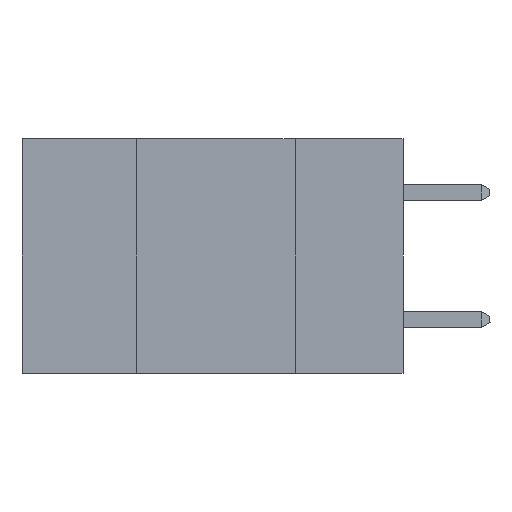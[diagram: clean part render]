
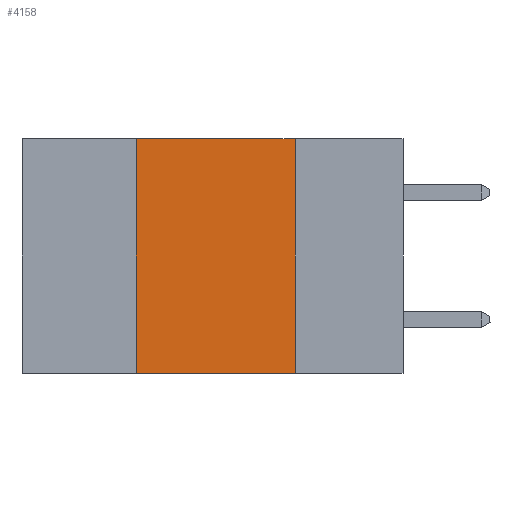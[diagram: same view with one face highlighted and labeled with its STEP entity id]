
A CAD part, left-side view. The second image highlights one B-rep face of the part: STEP entity #4158.
In plain terms, the highlighted planar face has unit normal (-1, 0, 0).
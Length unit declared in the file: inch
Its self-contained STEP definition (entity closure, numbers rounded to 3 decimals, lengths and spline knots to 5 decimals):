
#56 = VERTEX_POINT ( 'NONE', #4132 ) ;
#407 = ORIENTED_EDGE ( 'NONE', *, *, #18140, .F. ) ;
#415 = CARTESIAN_POINT ( 'NONE',  ( 0., 0.6, 0. ) ) ;
#479 = CARTESIAN_POINT ( 'NONE',  ( 0., 0.6, 0. ) ) ;
#500 = VERTEX_POINT ( 'NONE', #14114 ) ;
#1585 = LINE ( 'NONE', #24247, #8434 ) ;
#2094 = FACE_OUTER_BOUND ( 'NONE', #13984, .T. ) ;
#2759 = EDGE_CURVE ( 'NONE', #56, #4055, #1585, .T. ) ;
#3131 = CARTESIAN_POINT ( 'NONE',  ( 0., 0.17, -0.37 ) ) ;
#4055 = VERTEX_POINT ( 'NONE', #3131 ) ;
#4132 = CARTESIAN_POINT ( 'NONE',  ( 0., 0.42, -0.37 ) ) ;
#4158 = ADVANCED_FACE ( 'NONE', ( #2094 ), #17834, .F. ) ;
#6752 = EDGE_CURVE ( 'NONE', #16258, #500, #18745, .T. ) ;
#7124 = DIRECTION ( 'NONE',  ( 0., -1., 0. ) ) ;
#7333 = VECTOR ( 'NONE', #21498, 39.37008 ) ;
#8434 = VECTOR ( 'NONE', #7124, 39.37008 ) ;
#8459 = DIRECTION ( 'NONE',  ( 1., 0., 0. ) ) ;
#10269 = ORIENTED_EDGE ( 'NONE', *, *, #6752, .F. ) ;
#11099 = ORIENTED_EDGE ( 'NONE', *, *, #18207, .F. ) ;
#11165 = CARTESIAN_POINT ( 'NONE',  ( 0., 0.42, 0. ) ) ;
#11285 = LINE ( 'NONE', #13721, #15413 ) ;
#13721 = CARTESIAN_POINT ( 'NONE',  ( 0., 0.17, 0. ) ) ;
#13916 = ORIENTED_EDGE ( 'NONE', *, *, #2759, .T. ) ;
#13984 = EDGE_LOOP ( 'NONE', ( #407, #10269, #11099, #13916 ) ) ;
#14114 = CARTESIAN_POINT ( 'NONE',  ( 0., 0.17, 0. ) ) ;
#15413 = VECTOR ( 'NONE', #15632, 39.37008 ) ;
#15632 = DIRECTION ( 'NONE',  ( 0., 0., -1. ) ) ;
#16258 = VERTEX_POINT ( 'NONE', #11165 ) ;
#17834 = PLANE ( 'NONE',  #23418 ) ;
#18140 = EDGE_CURVE ( 'NONE', #500, #4055, #11285, .T. ) ;
#18207 = EDGE_CURVE ( 'NONE', #56, #16258, #24644, .T. ) ;
#18745 = LINE ( 'NONE', #415, #7333 ) ;
#19618 = VECTOR ( 'NONE', #19950, 39.37008 ) ;
#19950 = DIRECTION ( 'NONE',  ( 0., 0., 1. ) ) ;
#21498 = DIRECTION ( 'NONE',  ( 0., -1., 0. ) ) ;
#21769 = CARTESIAN_POINT ( 'NONE',  ( 0., 0.42, 0. ) ) ;
#21972 = DIRECTION ( 'NONE',  ( 0., 0., -1. ) ) ;
#23418 = AXIS2_PLACEMENT_3D ( 'NONE', #479, #8459, #21972 ) ;
#24247 = CARTESIAN_POINT ( 'NONE',  ( 0., 0.6, -0.37 ) ) ;
#24644 = LINE ( 'NONE', #21769, #19618 ) ;
